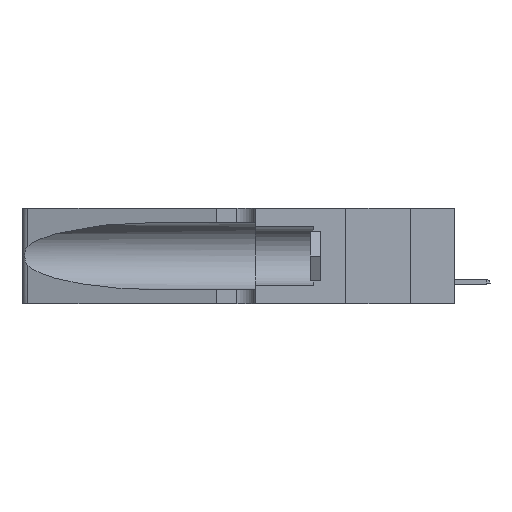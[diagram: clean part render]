
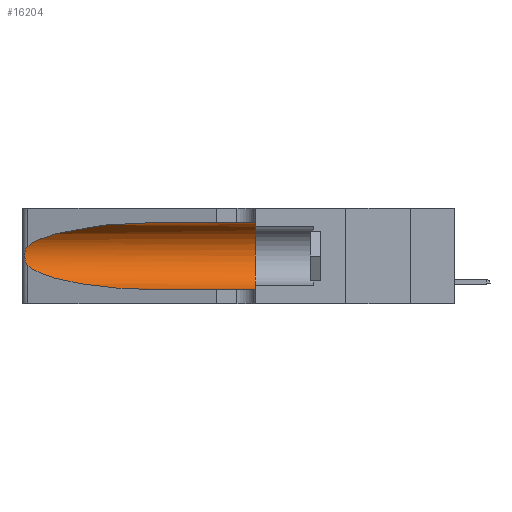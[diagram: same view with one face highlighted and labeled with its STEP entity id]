
A CAD part, left-side view. The second image highlights one B-rep face of the part: STEP entity #16204.
In plain terms, the highlighted cylindrical face has radius 3.308 mm (diameter 6.617 mm), a partial arc.
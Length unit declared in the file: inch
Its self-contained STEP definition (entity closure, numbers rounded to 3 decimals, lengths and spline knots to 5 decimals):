
#37 =( BOUNDED_CURVE ( )  B_SPLINE_CURVE ( 3, ( #822, #32712, #9048, #22190 ),
 .UNSPECIFIED., .F., .T. ) 
 B_SPLINE_CURVE_WITH_KNOTS ( ( 4, 4 ),
 ( 3.44316, 4.71239 ),
 .UNSPECIFIED. ) 
 CURVE ( )  GEOMETRIC_REPRESENTATION_ITEM ( )  RATIONAL_B_SPLINE_CURVE ( ( 1., 0.87, 0.87, 1. ) ) 
 REPRESENTATION_ITEM ( '' )  );
#739 = VERTEX_POINT ( 'NONE', #33624 ) ;
#822 = CARTESIAN_POINT ( 'NONE',  ( 0.25487, 1.22718, 0.14631 ) ) ;
#1181 = CARTESIAN_POINT ( 'NONE',  ( 0.25555, 1.22994, 0.2215 ) ) ;
#1290 = B_SPLINE_CURVE_WITH_KNOTS ( 'NONE', 3,
 ( #14787, #1181, #20072, #25361, #11994, #22369, #9234, #6762, #11821, #33246, #6595, #28175, #32891, #3809 ),
 .UNSPECIFIED., .F., .F.,
 ( 4, 2, 2, 2, 2, 2, 4 ),
 ( 0., 0.00027, 0.00053, 0.00107, 0.0016, 0.00187, 0.00214 ),
 .UNSPECIFIED. ) ;
#2313 = ORIENTED_EDGE ( 'NONE', *, *, #20196, .T. ) ;
#2366 = CARTESIAN_POINT ( 'NONE',  ( 0.1305, 0.72297, 0.05475 ) ) ;
#2472 = DIRECTION ( 'NONE',  ( 0., 1., 0. ) ) ;
#2860 = VERTEX_POINT ( 'NONE', #9710 ) ;
#3717 = VERTEX_POINT ( 'NONE', #2366 ) ;
#3809 = CARTESIAN_POINT ( 'NONE',  ( 0.25487, 1.22718, 0.14631 ) ) ;
#3814 = FACE_OUTER_BOUND ( 'NONE', #18884, .T. ) ;
#5713 = EDGE_CURVE ( 'NONE', #24661, #2860, #6689, .T. ) ;
#6595 = CARTESIAN_POINT ( 'NONE',  ( 0.25789, 1.23486, 0.15765 ) ) ;
#6689 = LINE ( 'NONE', #17336, #15115 ) ;
#6762 = CARTESIAN_POINT ( 'NONE',  ( 0.26075, 1.23896, 0.178 ) ) ;
#7123 = EDGE_CURVE ( 'NONE', #2860, #739, #26787, .T. ) ;
#8530 = CYLINDRICAL_SURFACE ( 'NONE', #30147, 0.13025 ) ;
#8700 = CARTESIAN_POINT ( 'NONE',  ( 0.25487, 1.22718, 0.22369 ) ) ;
#9048 = CARTESIAN_POINT ( 'NONE',  ( 0.18966, 0.96281, 0.05475 ) ) ;
#9063 = DIRECTION ( 'NONE',  ( 0., 0., -1. ) ) ;
#9234 = CARTESIAN_POINT ( 'NONE',  ( 0.26075, 1.23896, 0.19203 ) ) ;
#9710 = CARTESIAN_POINT ( 'NONE',  ( 0.1305, 0.35, 0.31525 ) ) ;
#10853 = DIRECTION ( 'NONE',  ( 0., -1., 0. ) ) ;
#11821 = CARTESIAN_POINT ( 'NONE',  ( 0.26017, 1.23833, 0.17102 ) ) ;
#11877 =( BOUNDED_CURVE ( )  B_SPLINE_CURVE ( 3, ( #33532, #33711, #25662, #17708 ),
 .UNSPECIFIED., .F., .F. ) 
 B_SPLINE_CURVE_WITH_KNOTS ( ( 4, 4 ),
 ( 1.5708, 2.84003 ),
 .UNSPECIFIED. ) 
 CURVE ( )  GEOMETRIC_REPRESENTATION_ITEM ( )  RATIONAL_B_SPLINE_CURVE ( ( 1., 0.87, 0.87, 1. ) ) 
 REPRESENTATION_ITEM ( '' )  );
#11994 = CARTESIAN_POINT ( 'NONE',  ( 0.25854, 1.2359, 0.20912 ) ) ;
#13638 = DIRECTION ( 'NONE',  ( 0., 0., 1. ) ) ;
#14787 = CARTESIAN_POINT ( 'NONE',  ( 0.25487, 1.22718, 0.22369 ) ) ;
#15115 = VECTOR ( 'NONE', #10853, 39.37008 ) ;
#15489 = CARTESIAN_POINT ( 'NONE',  ( 0.25487, 1.22718, 0.14631 ) ) ;
#16204 = ADVANCED_FACE ( 'NONE', ( #3814 ), #8530, .F. ) ;
#17336 = CARTESIAN_POINT ( 'NONE',  ( 0.1305, 1.61858, 0.31525 ) ) ;
#17708 = CARTESIAN_POINT ( 'NONE',  ( 0.25487, 1.22718, 0.22369 ) ) ;
#17939 = EDGE_CURVE ( 'NONE', #24661, #21190, #11877, .T. ) ;
#18884 = EDGE_LOOP ( 'NONE', ( #23913, #19299, #18933, #2313, #30055, #33364 ) ) ;
#18933 = ORIENTED_EDGE ( 'NONE', *, *, #28757, .T. ) ;
#19210 = CARTESIAN_POINT ( 'NONE',  ( 0.1305, 1.61858, 0.185 ) ) ;
#19299 = ORIENTED_EDGE ( 'NONE', *, *, #22657, .T. ) ;
#20065 = AXIS2_PLACEMENT_3D ( 'NONE', #29122, #2472, #13638 ) ;
#20072 = CARTESIAN_POINT ( 'NONE',  ( 0.25639, 1.23184, 0.21858 ) ) ;
#20196 = EDGE_CURVE ( 'NONE', #3717, #739, #23037, .T. ) ;
#20833 = VECTOR ( 'NONE', #28332, 39.37008 ) ;
#21190 = VERTEX_POINT ( 'NONE', #8700 ) ;
#22190 = CARTESIAN_POINT ( 'NONE',  ( 0.1305, 0.72297, 0.05475 ) ) ;
#22369 = CARTESIAN_POINT ( 'NONE',  ( 0.26018, 1.23835, 0.19895 ) ) ;
#22657 = EDGE_CURVE ( 'NONE', #21190, #33955, #1290, .T. ) ;
#23037 = LINE ( 'NONE', #30943, #20833 ) ;
#23913 = ORIENTED_EDGE ( 'NONE', *, *, #17939, .T. ) ;
#24661 = VERTEX_POINT ( 'NONE', #25598 ) ;
#25361 = CARTESIAN_POINT ( 'NONE',  ( 0.25787, 1.23484, 0.2124 ) ) ;
#25598 = CARTESIAN_POINT ( 'NONE',  ( 0.1305, 0.72297, 0.31525 ) ) ;
#25662 = CARTESIAN_POINT ( 'NONE',  ( 0.2373, 1.15595, 0.28018 ) ) ;
#26787 = CIRCLE ( 'NONE', #20065, 0.13025 ) ;
#28175 = CARTESIAN_POINT ( 'NONE',  ( 0.25639, 1.23186, 0.15144 ) ) ;
#28332 = DIRECTION ( 'NONE',  ( 0., -1., 0. ) ) ;
#28757 = EDGE_CURVE ( 'NONE', #33955, #3717, #37, .T. ) ;
#29122 = CARTESIAN_POINT ( 'NONE',  ( 0.1305, 0.35, 0.185 ) ) ;
#30055 = ORIENTED_EDGE ( 'NONE', *, *, #7123, .F. ) ;
#30147 = AXIS2_PLACEMENT_3D ( 'NONE', #19210, #33067, #9063 ) ;
#30943 = CARTESIAN_POINT ( 'NONE',  ( 0.1305, 1.61858, 0.05475 ) ) ;
#32712 = CARTESIAN_POINT ( 'NONE',  ( 0.2373, 1.15595, 0.08982 ) ) ;
#32891 = CARTESIAN_POINT ( 'NONE',  ( 0.25555, 1.22993, 0.14849 ) ) ;
#33067 = DIRECTION ( 'NONE',  ( 0., -1., 0. ) ) ;
#33246 = CARTESIAN_POINT ( 'NONE',  ( 0.25856, 1.23593, 0.16098 ) ) ;
#33364 = ORIENTED_EDGE ( 'NONE', *, *, #5713, .F. ) ;
#33532 = CARTESIAN_POINT ( 'NONE',  ( 0.1305, 0.72297, 0.31525 ) ) ;
#33624 = CARTESIAN_POINT ( 'NONE',  ( 0.1305, 0.35, 0.05475 ) ) ;
#33711 = CARTESIAN_POINT ( 'NONE',  ( 0.18966, 0.96281, 0.31525 ) ) ;
#33955 = VERTEX_POINT ( 'NONE', #15489 ) ;
